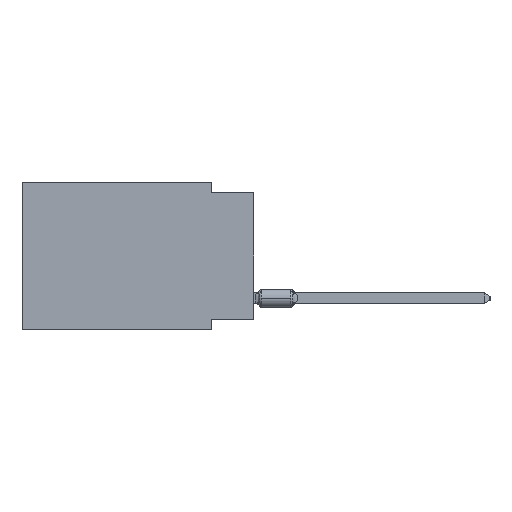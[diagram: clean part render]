
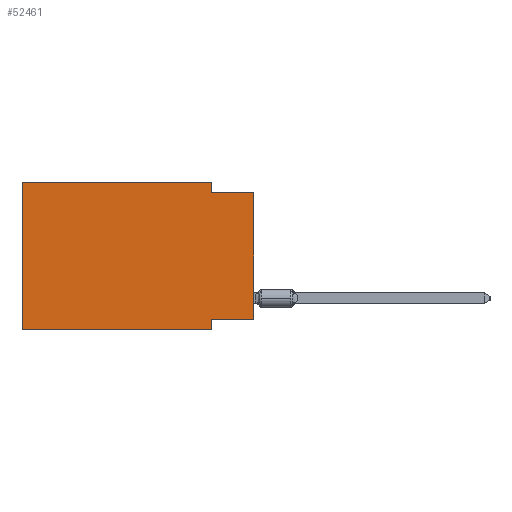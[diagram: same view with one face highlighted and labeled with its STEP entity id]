
A CAD part, left-side view. The second image highlights one B-rep face of the part: STEP entity #52461.
In plain terms, the highlighted planar face has unit normal (-1, 0, 0).
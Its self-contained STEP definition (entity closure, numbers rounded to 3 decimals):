
#157 = VECTOR ( 'NONE', #50631, 1000. ) ;
#1488 = VECTOR ( 'NONE', #5213, 1000. ) ;
#2741 = EDGE_CURVE ( 'NONE', #6717, #47232, #7940, .T. ) ;
#3677 = ORIENTED_EDGE ( 'NONE', *, *, #37202, .F. ) ;
#5213 = DIRECTION ( 'NONE',  ( 0., 0., -1. ) ) ;
#6717 = VERTEX_POINT ( 'NONE', #74694 ) ;
#7940 = LINE ( 'NONE', #42922, #12636 ) ;
#9269 = CARTESIAN_POINT ( 'NONE',  ( 0., 13.97, 0. ) ) ;
#9813 = VERTEX_POINT ( 'NONE', #15365 ) ;
#10810 = CARTESIAN_POINT ( 'NONE',  ( 0., 0., -8.255 ) ) ;
#11032 = CARTESIAN_POINT ( 'NONE',  ( 0., 2.54, -8.89 ) ) ;
#12035 = CARTESIAN_POINT ( 'NONE',  ( 0., 2.54, -8.89 ) ) ;
#12636 = VECTOR ( 'NONE', #55360, 1000. ) ;
#15021 = VERTEX_POINT ( 'NONE', #67497 ) ;
#15365 = CARTESIAN_POINT ( 'NONE',  ( 0., 0., -8.255 ) ) ;
#16871 = LINE ( 'NONE', #11032, #1488 ) ;
#19381 = VECTOR ( 'NONE', #61409, 1000. ) ;
#19435 = LINE ( 'NONE', #10810, #46218 ) ;
#23376 = LINE ( 'NONE', #51795, #25016 ) ;
#23626 = CARTESIAN_POINT ( 'NONE',  ( 0., 13.97, -8.89 ) ) ;
#23885 = EDGE_CURVE ( 'NONE', #50132, #56857, #38551, .T. ) ;
#24025 = EDGE_CURVE ( 'NONE', #9813, #47232, #23376, .T. ) ;
#25016 = VECTOR ( 'NONE', #52563, 1000. ) ;
#25185 = ORIENTED_EDGE ( 'NONE', *, *, #24025, .T. ) ;
#25630 = CARTESIAN_POINT ( 'NONE',  ( 0., 2.54, 0. ) ) ;
#27302 = ORIENTED_EDGE ( 'NONE', *, *, #35157, .F. ) ;
#32979 = DIRECTION ( 'NONE',  ( 0., -1., 0. ) ) ;
#33945 = DIRECTION ( 'NONE',  ( 1., 0., 0. ) ) ;
#35157 = EDGE_CURVE ( 'NONE', #9813, #15021, #19435, .T. ) ;
#35253 = DIRECTION ( 'NONE',  ( 0., 1., 0. ) ) ;
#37202 = EDGE_CURVE ( 'NONE', #51158, #58010, #38787, .T. ) ;
#37915 = VECTOR ( 'NONE', #68392, 1000. ) ;
#38551 = LINE ( 'NONE', #56084, #157 ) ;
#38787 = LINE ( 'NONE', #9269, #65055 ) ;
#40051 = CARTESIAN_POINT ( 'NONE',  ( 0., 2.54, 0. ) ) ;
#42329 = CARTESIAN_POINT ( 'NONE',  ( 0., 13.97, 0. ) ) ;
#42922 = CARTESIAN_POINT ( 'NONE',  ( 0., 0., -0.635 ) ) ;
#45596 = PLANE ( 'NONE',  #52913 ) ;
#46218 = VECTOR ( 'NONE', #35253, 1000. ) ;
#47232 = VERTEX_POINT ( 'NONE', #64922 ) ;
#48567 = LINE ( 'NONE', #25630, #19381 ) ;
#49565 = ORIENTED_EDGE ( 'NONE', *, *, #23885, .T. ) ;
#50068 = EDGE_CURVE ( 'NONE', #50132, #51158, #63725, .T. ) ;
#50132 = VERTEX_POINT ( 'NONE', #23626 ) ;
#50631 = DIRECTION ( 'NONE',  ( 0., -1., 0. ) ) ;
#51158 = VERTEX_POINT ( 'NONE', #42329 ) ;
#51795 = CARTESIAN_POINT ( 'NONE',  ( 0., 0., 0. ) ) ;
#52328 = ORIENTED_EDGE ( 'NONE', *, *, #2741, .F. ) ;
#52355 = ORIENTED_EDGE ( 'NONE', *, *, #52590, .F. ) ;
#52461 = ADVANCED_FACE ( 'NONE', ( #75563 ), #45596, .F. ) ;
#52529 = ORIENTED_EDGE ( 'NONE', *, *, #54924, .F. ) ;
#52563 = DIRECTION ( 'NONE',  ( 0., 0., 1. ) ) ;
#52590 = EDGE_CURVE ( 'NONE', #58010, #6717, #48567, .T. ) ;
#52913 = AXIS2_PLACEMENT_3D ( 'NONE', #54041, #33945, #71552 ) ;
#54041 = CARTESIAN_POINT ( 'NONE',  ( 0., 13.97, 0. ) ) ;
#54924 = EDGE_CURVE ( 'NONE', #15021, #56857, #16871, .T. ) ;
#55360 = DIRECTION ( 'NONE',  ( 0., -1., 0. ) ) ;
#56084 = CARTESIAN_POINT ( 'NONE',  ( 0., 13.97, -8.89 ) ) ;
#56857 = VERTEX_POINT ( 'NONE', #12035 ) ;
#58010 = VERTEX_POINT ( 'NONE', #40051 ) ;
#58253 = EDGE_LOOP ( 'NONE', ( #25185, #52328, #52355, #3677, #75671, #49565, #52529, #27302 ) ) ;
#61409 = DIRECTION ( 'NONE',  ( 0., 0., -1. ) ) ;
#63725 = LINE ( 'NONE', #73851, #37915 ) ;
#64922 = CARTESIAN_POINT ( 'NONE',  ( 0., 0., -0.635 ) ) ;
#65055 = VECTOR ( 'NONE', #32979, 1000. ) ;
#67497 = CARTESIAN_POINT ( 'NONE',  ( 0., 2.54, -8.255 ) ) ;
#68392 = DIRECTION ( 'NONE',  ( 0., 0., 1. ) ) ;
#71552 = DIRECTION ( 'NONE',  ( 0., 0., -1. ) ) ;
#73851 = CARTESIAN_POINT ( 'NONE',  ( 0., 13.97, 0. ) ) ;
#74694 = CARTESIAN_POINT ( 'NONE',  ( 0., 2.54, -0.635 ) ) ;
#75563 = FACE_OUTER_BOUND ( 'NONE', #58253, .T. ) ;
#75671 = ORIENTED_EDGE ( 'NONE', *, *, #50068, .F. ) ;
